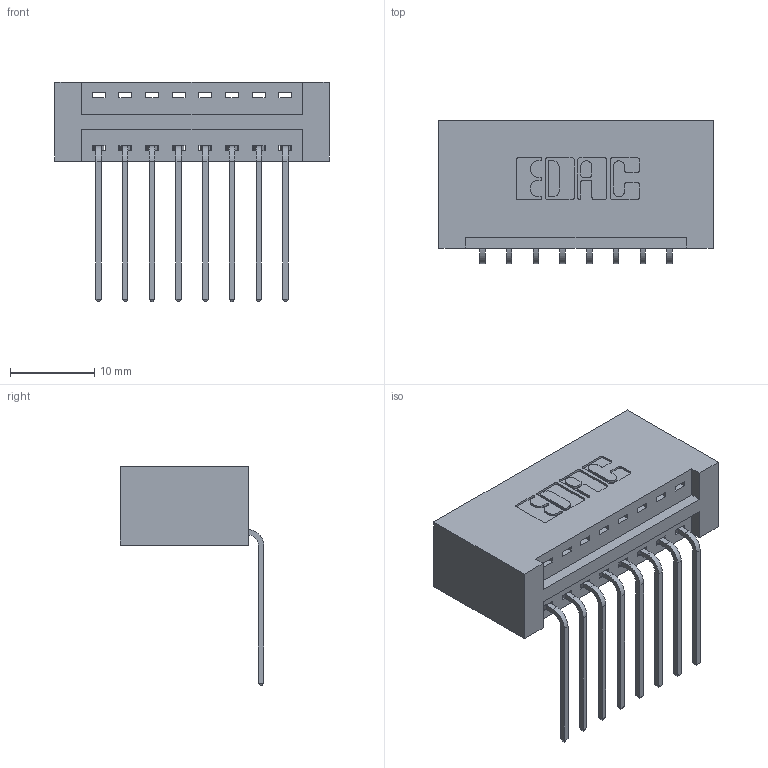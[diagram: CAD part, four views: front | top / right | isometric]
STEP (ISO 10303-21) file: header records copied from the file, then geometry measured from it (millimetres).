
FILE_DESCRIPTION (( 'STEP AP203' ), '1' );
FILE_NAME ('346-008-559-101.STEP', '2022-05-04T21:38:15', ( '' ), ( '' ), 'SwSTEP 2.0', 'SolidWorks 2020', '' );
FILE_SCHEMA (( 'CONFIG_CONTROL_DESIGN' ));
Length unit declared in the file: inch
Products named in the file (3): 346 Part_No Mounting Lugs; 345-292-001_558 559 Tail - 1; 346-008-559-101
Assembly tree (9 placements, depth 2):
  346-008-559-101
    346 Part_No Mounting Lugs
    345-292-001_558 559 Tail - 1  x8
Bounding box: 32.64 x 17.08 x 26.16 mm (x, y, z)
Volume: 3466.1 mm3; surface area: 4199.4 mm2
Topology: 9 solids, 9 shells, 594 faces, 1761 edges, 1162 vertices
Faces by surface type: plane 408, cylinder 186
Entity records: 9349 total; most frequent: CARTESIAN_POINT 1620, ORIENTED_EDGE 1562, DIRECTION 1465, EDGE_CURVE 781, LINE 625, VECTOR 625, VERTEX_POINT 518, AXIS2_PLACEMENT_3D 420
